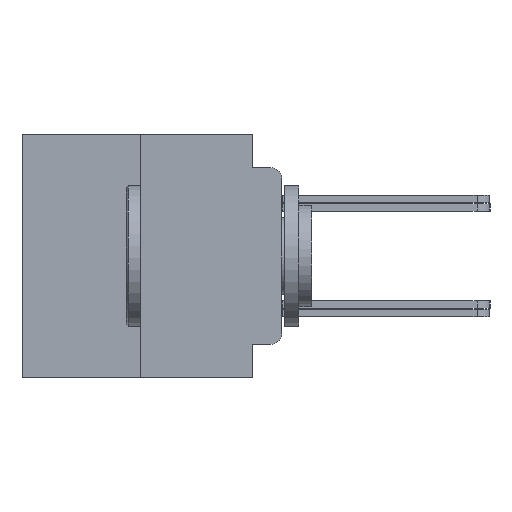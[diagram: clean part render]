
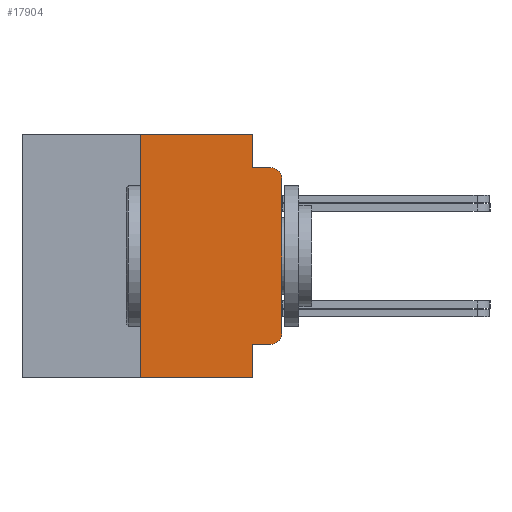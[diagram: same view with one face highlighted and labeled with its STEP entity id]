
A CAD part, left-side view. The second image highlights one B-rep face of the part: STEP entity #17904.
In plain terms, the highlighted planar face has unit normal (-1, 0, 0).
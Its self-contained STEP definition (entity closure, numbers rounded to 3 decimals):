
#283 = DIRECTION ( 'NONE',  ( 1., 0., 0. ) ) ;
#684 = CARTESIAN_POINT ( 'NONE',  ( -75.603, 0.508, -3.467 ) ) ;
#781 = CARTESIAN_POINT ( 'NONE',  ( -75.603, 0.508, 3.467 ) ) ;
#858 = DIRECTION ( 'NONE',  ( 0., 0., 1. ) ) ;
#991 = VECTOR ( 'NONE', #24385, 1000. ) ;
#1044 = CARTESIAN_POINT ( 'NONE',  ( -75.603, 0., 3.467 ) ) ;
#1807 = LINE ( 'NONE', #12756, #25417 ) ;
#1882 = VERTEX_POINT ( 'NONE', #22704 ) ;
#2463 = CARTESIAN_POINT ( 'NONE',  ( -75.603, 6.35, 5.486 ) ) ;
#4051 = DIRECTION ( 'NONE',  ( 0., -1., 0. ) ) ;
#4095 = ORIENTED_EDGE ( 'NONE', *, *, #7793, .F. ) ;
#4497 = VERTEX_POINT ( 'NONE', #7410 ) ;
#5278 = DIRECTION ( 'NONE',  ( 0., 0., -1. ) ) ;
#6252 = ORIENTED_EDGE ( 'NONE', *, *, #26147, .F. ) ;
#7356 = EDGE_CURVE ( 'NONE', #25251, #12286, #26424, .T. ) ;
#7410 = CARTESIAN_POINT ( 'NONE',  ( -75.603, 0.508, -3.975 ) ) ;
#7513 = CARTESIAN_POINT ( 'NONE',  ( -75.603, 6.35, -5.486 ) ) ;
#7596 = ORIENTED_EDGE ( 'NONE', *, *, #12463, .F. ) ;
#7793 = EDGE_CURVE ( 'NONE', #13952, #1882, #17792, .T. ) ;
#8291 = VERTEX_POINT ( 'NONE', #12721 ) ;
#8342 = DIRECTION ( 'NONE',  ( 0., -1., 0. ) ) ;
#8359 = CARTESIAN_POINT ( 'NONE',  ( -75.603, 11.684, 5.486 ) ) ;
#8745 = CARTESIAN_POINT ( 'NONE',  ( -75.603, 1.295, -3.975 ) ) ;
#9188 = VECTOR ( 'NONE', #858, 1000. ) ;
#9553 = AXIS2_PLACEMENT_3D ( 'NONE', #781, #19080, #28887 ) ;
#10058 = DIRECTION ( 'NONE',  ( 0., 0., -1. ) ) ;
#10491 = VECTOR ( 'NONE', #27933, 1000. ) ;
#11076 = FACE_OUTER_BOUND ( 'NONE', #20621, .T. ) ;
#11153 = LINE ( 'NONE', #22140, #25474 ) ;
#11329 = CIRCLE ( 'NONE', #16495, 0.508 ) ;
#11698 = ORIENTED_EDGE ( 'NONE', *, *, #7356, .T. ) ;
#12286 = VERTEX_POINT ( 'NONE', #15214 ) ;
#12387 = ORIENTED_EDGE ( 'NONE', *, *, #19610, .F. ) ;
#12463 = EDGE_CURVE ( 'NONE', #27849, #8291, #25188, .T. ) ;
#12721 = CARTESIAN_POINT ( 'NONE',  ( -75.603, 1.295, 3.975 ) ) ;
#12756 = CARTESIAN_POINT ( 'NONE',  ( -75.603, 11.684, -5.486 ) ) ;
#13388 = LINE ( 'NONE', #7513, #10491 ) ;
#13738 = ORIENTED_EDGE ( 'NONE', *, *, #22041, .F. ) ;
#13952 = VERTEX_POINT ( 'NONE', #17200 ) ;
#14699 = EDGE_CURVE ( 'NONE', #21458, #1882, #1807, .T. ) ;
#15214 = CARTESIAN_POINT ( 'NONE',  ( -75.603, 0.508, 3.975 ) ) ;
#16012 = CARTESIAN_POINT ( 'NONE',  ( -75.603, 11.684, 5.486 ) ) ;
#16022 = VECTOR ( 'NONE', #4051, 1000. ) ;
#16137 = ORIENTED_EDGE ( 'NONE', *, *, #19720, .T. ) ;
#16495 = AXIS2_PLACEMENT_3D ( 'NONE', #684, #19392, #10058 ) ;
#16822 = CARTESIAN_POINT ( 'NONE',  ( -75.603, 1.295, 5.486 ) ) ;
#16982 = CARTESIAN_POINT ( 'NONE',  ( -75.603, 6.35, -5.486 ) ) ;
#17200 = CARTESIAN_POINT ( 'NONE',  ( -75.603, 1.295, -3.975 ) ) ;
#17264 = CARTESIAN_POINT ( 'NONE',  ( -75.603, 0., -3.467 ) ) ;
#17792 = LINE ( 'NONE', #21010, #21020 ) ;
#17904 = ADVANCED_FACE ( 'NONE', ( #11076 ), #18270, .F. ) ;
#17915 = VERTEX_POINT ( 'NONE', #2463 ) ;
#18146 = LINE ( 'NONE', #8359, #991 ) ;
#18270 = PLANE ( 'NONE',  #29508 ) ;
#18855 = ORIENTED_EDGE ( 'NONE', *, *, #19446, .T. ) ;
#19080 = DIRECTION ( 'NONE',  ( -1., 0., 0. ) ) ;
#19392 = DIRECTION ( 'NONE',  ( -1., 0., 0. ) ) ;
#19446 = EDGE_CURVE ( 'NONE', #4497, #22819, #11329, .T. ) ;
#19610 = EDGE_CURVE ( 'NONE', #17915, #27849, #18146, .T. ) ;
#19720 = EDGE_CURVE ( 'NONE', #13952, #4497, #24921, .T. ) ;
#20311 = LINE ( 'NONE', #28361, #9188 ) ;
#20621 = EDGE_LOOP ( 'NONE', ( #16137, #18855, #27697, #11698, #6252, #7596, #12387, #13738, #26483, #4095 ) ) ;
#21010 = CARTESIAN_POINT ( 'NONE',  ( -75.603, 1.295, 0. ) ) ;
#21020 = VECTOR ( 'NONE', #25593, 1000. ) ;
#21458 = VERTEX_POINT ( 'NONE', #16982 ) ;
#21941 = DIRECTION ( 'NONE',  ( 0., -1., 0. ) ) ;
#22041 = EDGE_CURVE ( 'NONE', #21458, #17915, #13388, .T. ) ;
#22140 = CARTESIAN_POINT ( 'NONE',  ( -75.603, 1.295, 3.975 ) ) ;
#22686 = EDGE_CURVE ( 'NONE', #22819, #25251, #20311, .T. ) ;
#22704 = CARTESIAN_POINT ( 'NONE',  ( -75.603, 1.295, -5.486 ) ) ;
#22819 = VERTEX_POINT ( 'NONE', #17264 ) ;
#22918 = DIRECTION ( 'NONE',  ( 0., 0., -1. ) ) ;
#23410 = CARTESIAN_POINT ( 'NONE',  ( -75.603, 1.295, 0. ) ) ;
#24385 = DIRECTION ( 'NONE',  ( 0., -1., 0. ) ) ;
#24921 = LINE ( 'NONE', #8745, #16022 ) ;
#25188 = LINE ( 'NONE', #23410, #25562 ) ;
#25251 = VERTEX_POINT ( 'NONE', #1044 ) ;
#25417 = VECTOR ( 'NONE', #8342, 1000. ) ;
#25474 = VECTOR ( 'NONE', #21941, 1000. ) ;
#25562 = VECTOR ( 'NONE', #5278, 1000. ) ;
#25593 = DIRECTION ( 'NONE',  ( 0., 0., -1. ) ) ;
#26147 = EDGE_CURVE ( 'NONE', #8291, #12286, #11153, .T. ) ;
#26424 = CIRCLE ( 'NONE', #9553, 0.508 ) ;
#26483 = ORIENTED_EDGE ( 'NONE', *, *, #14699, .T. ) ;
#27697 = ORIENTED_EDGE ( 'NONE', *, *, #22686, .T. ) ;
#27849 = VERTEX_POINT ( 'NONE', #16822 ) ;
#27933 = DIRECTION ( 'NONE',  ( 0., 0., 1. ) ) ;
#28361 = CARTESIAN_POINT ( 'NONE',  ( -75.603, 0., 5.486 ) ) ;
#28887 = DIRECTION ( 'NONE',  ( 0., 0., -1. ) ) ;
#29508 = AXIS2_PLACEMENT_3D ( 'NONE', #16012, #283, #22918 ) ;
